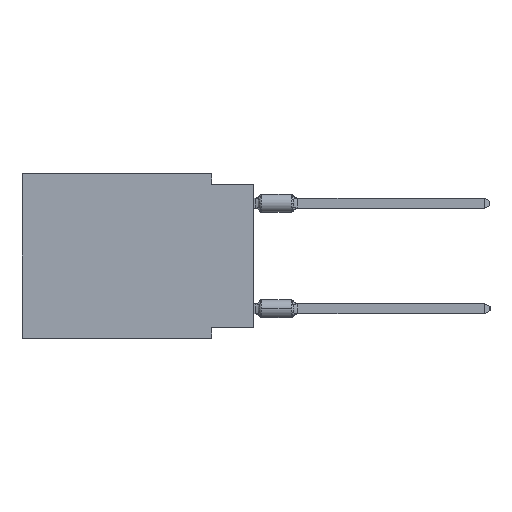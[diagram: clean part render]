
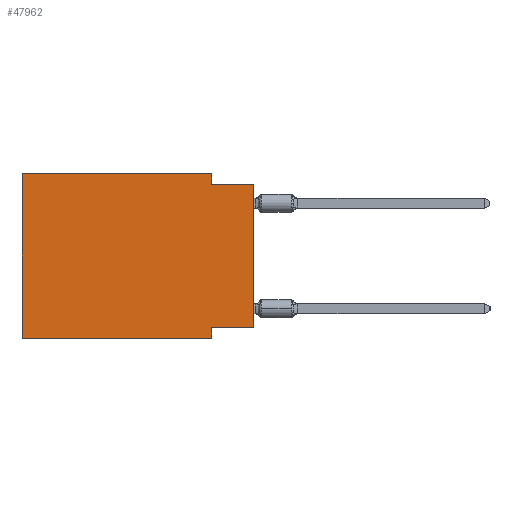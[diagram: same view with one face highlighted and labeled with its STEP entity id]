
A CAD part, left-side view. The second image highlights one B-rep face of the part: STEP entity #47962.
In plain terms, the highlighted planar face has unit normal (-1, 0, 0).
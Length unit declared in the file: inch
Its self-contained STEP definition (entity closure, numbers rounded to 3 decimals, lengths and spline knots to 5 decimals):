
#687 = ORIENTED_EDGE ( 'NONE', *, *, #52917, .F. ) ;
#1025 = VERTEX_POINT ( 'NONE', #12839 ) ;
#2897 = ORIENTED_EDGE ( 'NONE', *, *, #32912, .T. ) ;
#3520 = VECTOR ( 'NONE', #7268, 39.37008 ) ;
#3749 = VERTEX_POINT ( 'NONE', #27585 ) ;
#4401 = LINE ( 'NONE', #49681, #16083 ) ;
#6321 = VERTEX_POINT ( 'NONE', #24496 ) ;
#7268 = DIRECTION ( 'NONE',  ( 0., 0., -1. ) ) ;
#9625 = LINE ( 'NONE', #50679, #31985 ) ;
#10464 = LINE ( 'NONE', #13739, #25017 ) ;
#12207 = EDGE_CURVE ( 'NONE', #55305, #6321, #45696, .T. ) ;
#12839 = CARTESIAN_POINT ( 'NONE',  ( 0., 0., -0.365 ) ) ;
#13739 = CARTESIAN_POINT ( 'NONE',  ( 0., 0.55, 0. ) ) ;
#14563 = CARTESIAN_POINT ( 'NONE',  ( 0., 0.1, 0. ) ) ;
#16083 = VECTOR ( 'NONE', #17886, 39.37008 ) ;
#17723 = CARTESIAN_POINT ( 'NONE',  ( 0., 0., -0.365 ) ) ;
#17885 = ORIENTED_EDGE ( 'NONE', *, *, #35067, .F. ) ;
#17886 = DIRECTION ( 'NONE',  ( 0., 0., 1. ) ) ;
#20004 = LINE ( 'NONE', #33518, #39735 ) ;
#21087 = CARTESIAN_POINT ( 'NONE',  ( 0., 0.1, -0.365 ) ) ;
#22283 = VERTEX_POINT ( 'NONE', #34181 ) ;
#22476 = EDGE_CURVE ( 'NONE', #3749, #58791, #53970, .T. ) ;
#24496 = CARTESIAN_POINT ( 'NONE',  ( 0., 0.1, -0.39 ) ) ;
#25017 = VECTOR ( 'NONE', #32630, 39.37008 ) ;
#25924 = EDGE_CURVE ( 'NONE', #1025, #55305, #26706, .T. ) ;
#26706 = LINE ( 'NONE', #17723, #31656 ) ;
#27585 = CARTESIAN_POINT ( 'NONE',  ( 0., 0.1, -0.025 ) ) ;
#27746 = ORIENTED_EDGE ( 'NONE', *, *, #12207, .F. ) ;
#27986 = DIRECTION ( 'NONE',  ( 0., 0., 1. ) ) ;
#28372 = DIRECTION ( 'NONE',  ( 0., 0., -1. ) ) ;
#28433 = DIRECTION ( 'NONE',  ( 0., -1., 0. ) ) ;
#29430 = VERTEX_POINT ( 'NONE', #14563 ) ;
#30574 = CARTESIAN_POINT ( 'NONE',  ( 0., 0., -0.025 ) ) ;
#31528 = VECTOR ( 'NONE', #39584, 39.37008 ) ;
#31656 = VECTOR ( 'NONE', #36020, 39.37008 ) ;
#31985 = VECTOR ( 'NONE', #53990, 39.37008 ) ;
#32522 = VERTEX_POINT ( 'NONE', #44527 ) ;
#32630 = DIRECTION ( 'NONE',  ( 0., -1., 0. ) ) ;
#32912 = EDGE_CURVE ( 'NONE', #32522, #6321, #20004, .T. ) ;
#33169 = CARTESIAN_POINT ( 'NONE',  ( 0., 0.55, 0. ) ) ;
#33518 = CARTESIAN_POINT ( 'NONE',  ( 0., 0.55, -0.39 ) ) ;
#34181 = CARTESIAN_POINT ( 'NONE',  ( 0., 0.55, 0. ) ) ;
#34721 = ORIENTED_EDGE ( 'NONE', *, *, #35669, .T. ) ;
#35067 = EDGE_CURVE ( 'NONE', #32522, #22283, #37581, .T. ) ;
#35669 = EDGE_CURVE ( 'NONE', #1025, #58791, #4401, .T. ) ;
#36020 = DIRECTION ( 'NONE',  ( 0., 1., 0. ) ) ;
#36069 = AXIS2_PLACEMENT_3D ( 'NONE', #33169, #47551, #28372 ) ;
#36728 = EDGE_LOOP ( 'NONE', ( #34721, #55334, #687, #40396, #17885, #2897, #27746, #40397 ) ) ;
#37581 = LINE ( 'NONE', #37885, #50456 ) ;
#37885 = CARTESIAN_POINT ( 'NONE',  ( 0., 0.55, 0. ) ) ;
#37960 = PLANE ( 'NONE',  #36069 ) ;
#39584 = DIRECTION ( 'NONE',  ( 0., -1., 0. ) ) ;
#39735 = VECTOR ( 'NONE', #28433, 39.37008 ) ;
#40396 = ORIENTED_EDGE ( 'NONE', *, *, #42145, .F. ) ;
#40397 = ORIENTED_EDGE ( 'NONE', *, *, #25924, .F. ) ;
#42145 = EDGE_CURVE ( 'NONE', #22283, #29430, #10464, .T. ) ;
#44527 = CARTESIAN_POINT ( 'NONE',  ( 0., 0.55, -0.39 ) ) ;
#45696 = LINE ( 'NONE', #52528, #3520 ) ;
#47551 = DIRECTION ( 'NONE',  ( 1., 0., 0. ) ) ;
#47962 = ADVANCED_FACE ( 'NONE', ( #55372 ), #37960, .F. ) ;
#48467 = CARTESIAN_POINT ( 'NONE',  ( 0., 0., -0.025 ) ) ;
#49681 = CARTESIAN_POINT ( 'NONE',  ( 0., 0., 0. ) ) ;
#50456 = VECTOR ( 'NONE', #27986, 39.37008 ) ;
#50679 = CARTESIAN_POINT ( 'NONE',  ( 0., 0.1, 0. ) ) ;
#52528 = CARTESIAN_POINT ( 'NONE',  ( 0., 0.1, -0.39 ) ) ;
#52917 = EDGE_CURVE ( 'NONE', #29430, #3749, #9625, .T. ) ;
#53970 = LINE ( 'NONE', #30574, #31528 ) ;
#53990 = DIRECTION ( 'NONE',  ( 0., 0., -1. ) ) ;
#55305 = VERTEX_POINT ( 'NONE', #21087 ) ;
#55334 = ORIENTED_EDGE ( 'NONE', *, *, #22476, .F. ) ;
#55372 = FACE_OUTER_BOUND ( 'NONE', #36728, .T. ) ;
#58791 = VERTEX_POINT ( 'NONE', #48467 ) ;
